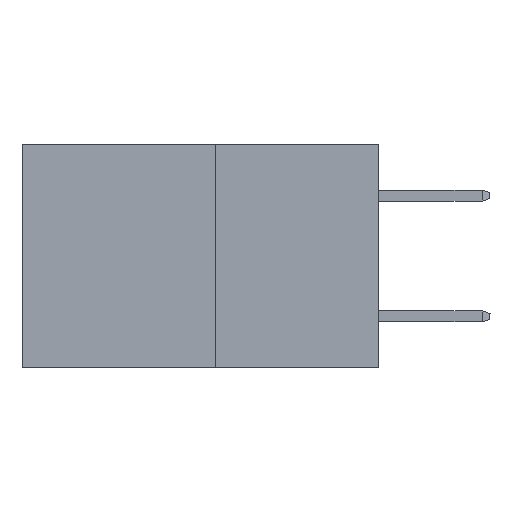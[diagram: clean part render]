
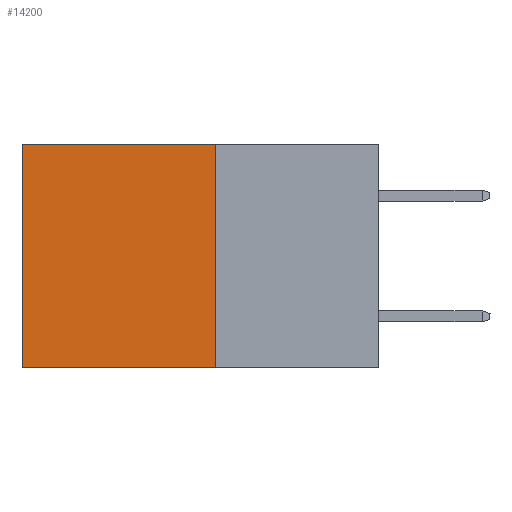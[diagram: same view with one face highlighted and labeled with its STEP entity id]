
A CAD part, left-side view. The second image highlights one B-rep face of the part: STEP entity #14200.
In plain terms, the highlighted planar face has unit normal (-1, 0, 0).
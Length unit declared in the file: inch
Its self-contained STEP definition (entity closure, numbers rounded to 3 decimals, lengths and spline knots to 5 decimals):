
#139 = EDGE_CURVE ( 'NONE', #11657, #9296, #5428, .T. ) ;
#468 = DIRECTION ( 'NONE',  ( 0., 0., -1. ) ) ;
#514 = PLANE ( 'NONE',  #25031 ) ;
#1652 = LINE ( 'NONE', #21977, #27328 ) ;
#1786 = CARTESIAN_POINT ( 'NONE',  ( 0.277, 0.59, 0. ) ) ;
#2391 = CARTESIAN_POINT ( 'NONE',  ( 0.277, 0.27, 0. ) ) ;
#2800 = LINE ( 'NONE', #17475, #8840 ) ;
#2943 = CARTESIAN_POINT ( 'NONE',  ( 0.277, 0.59, -0.37 ) ) ;
#5428 = LINE ( 'NONE', #6825, #31073 ) ;
#5702 = DIRECTION ( 'NONE',  ( 1., 0., 0. ) ) ;
#6260 = VECTOR ( 'NONE', #468, 39.37008 ) ;
#6825 = CARTESIAN_POINT ( 'NONE',  ( 0.277, 0.27, -0.37 ) ) ;
#8840 = VECTOR ( 'NONE', #22516, 39.37008 ) ;
#9296 = VERTEX_POINT ( 'NONE', #18992 ) ;
#9423 = CARTESIAN_POINT ( 'NONE',  ( 0.277, 0.59, -0.37 ) ) ;
#9502 = EDGE_LOOP ( 'NONE', ( #17997, #22129, #24908, #32949 ) ) ;
#11657 = VERTEX_POINT ( 'NONE', #2391 ) ;
#11959 = EDGE_CURVE ( 'NONE', #11657, #13877, #2800, .T. ) ;
#13044 = LINE ( 'NONE', #2943, #6260 ) ;
#13877 = VERTEX_POINT ( 'NONE', #1786 ) ;
#14200 = ADVANCED_FACE ( 'NONE', ( #21944 ), #514, .F. ) ;
#17475 = CARTESIAN_POINT ( 'NONE',  ( 0.277, 0.27, 0. ) ) ;
#17560 = EDGE_CURVE ( 'NONE', #13877, #31121, #13044, .T. ) ;
#17997 = ORIENTED_EDGE ( 'NONE', *, *, #17560, .T. ) ;
#18992 = CARTESIAN_POINT ( 'NONE',  ( 0.277, 0.27, -0.37 ) ) ;
#20949 = CARTESIAN_POINT ( 'NONE',  ( 0.277, 0.27, -0.37 ) ) ;
#21944 = FACE_OUTER_BOUND ( 'NONE', #9502, .T. ) ;
#21977 = CARTESIAN_POINT ( 'NONE',  ( 0.277, 0.27, -0.37 ) ) ;
#22129 = ORIENTED_EDGE ( 'NONE', *, *, #26363, .F. ) ;
#22516 = DIRECTION ( 'NONE',  ( 0., 1., 0. ) ) ;
#23297 = DIRECTION ( 'NONE',  ( 0., 0., -1. ) ) ;
#23645 = DIRECTION ( 'NONE',  ( 0., 0., -1. ) ) ;
#24586 = DIRECTION ( 'NONE',  ( 0., 1., 0. ) ) ;
#24908 = ORIENTED_EDGE ( 'NONE', *, *, #139, .F. ) ;
#25031 = AXIS2_PLACEMENT_3D ( 'NONE', #20949, #5702, #23645 ) ;
#26363 = EDGE_CURVE ( 'NONE', #9296, #31121, #1652, .T. ) ;
#27328 = VECTOR ( 'NONE', #24586, 39.37008 ) ;
#31073 = VECTOR ( 'NONE', #23297, 39.37008 ) ;
#31121 = VERTEX_POINT ( 'NONE', #9423 ) ;
#32949 = ORIENTED_EDGE ( 'NONE', *, *, #11959, .T. ) ;
